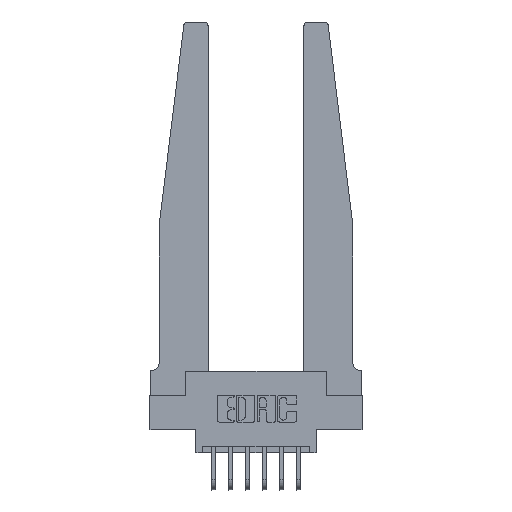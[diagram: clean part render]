
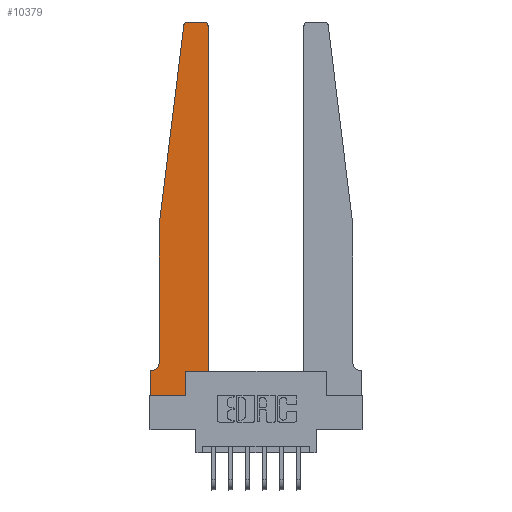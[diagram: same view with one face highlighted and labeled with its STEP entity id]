
A CAD part, top view. The second image highlights one B-rep face of the part: STEP entity #10379.
In plain terms, the highlighted planar face has unit normal (0, 0, 1).
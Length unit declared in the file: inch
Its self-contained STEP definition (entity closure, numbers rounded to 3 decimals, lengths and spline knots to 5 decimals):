
#15 = EDGE_CURVE ( 'NONE', #51, #5024, #1532, .T. ) ;
#51 = VERTEX_POINT ( 'NONE', #466 ) ;
#75 = DIRECTION ( 'NONE',  ( 0., 0., 1. ) ) ;
#79 = AXIS2_PLACEMENT_3D ( 'NONE', #8297, #8222, #9416 ) ;
#265 = DIRECTION ( 'NONE',  ( 0., -1., 0. ) ) ;
#386 = CARTESIAN_POINT ( 'NONE',  ( 0., 0.1875, 0.37 ) ) ;
#466 = CARTESIAN_POINT ( 'NONE',  ( 0.425, 0.18, 0.37 ) ) ;
#629 = LINE ( 'NONE', #7001, #10541 ) ;
#1075 = VECTOR ( 'NONE', #4248, 39.37008 ) ;
#1297 = AXIS2_PLACEMENT_3D ( 'NONE', #386, #4987, #5820 ) ;
#1425 = VERTEX_POINT ( 'NONE', #1536 ) ;
#1460 = EDGE_CURVE ( 'NONE', #2933, #8866, #4866, .T. ) ;
#1509 = VECTOR ( 'NONE', #9149, 39.37008 ) ;
#1532 = LINE ( 'NONE', #10071, #1509 ) ;
#1536 = CARTESIAN_POINT ( 'NONE',  ( 0.2605, 0., 0.37 ) ) ;
#1804 = CARTESIAN_POINT ( 'NONE',  ( 0.395, 2.75, 0.37 ) ) ;
#2175 = ORIENTED_EDGE ( 'NONE', *, *, #1460, .T. ) ;
#2325 = DIRECTION ( 'NONE',  ( 1., 0., 0. ) ) ;
#2933 = VERTEX_POINT ( 'NONE', #6547 ) ;
#3113 = DIRECTION ( 'NONE',  ( 1., 0., 0. ) ) ;
#3441 = EDGE_CURVE ( 'NONE', #8767, #4837, #9859, .T. ) ;
#3532 = VERTEX_POINT ( 'NONE', #3998 ) ;
#3546 = ORIENTED_EDGE ( 'NONE', *, *, #7056, .T. ) ;
#3662 = VECTOR ( 'NONE', #10256, 39.37008 ) ;
#3867 = DIRECTION ( 'NONE',  ( -1., 0., 0. ) ) ;
#3877 = VERTEX_POINT ( 'NONE', #13833 ) ;
#3893 = ORIENTED_EDGE ( 'NONE', *, *, #12143, .T. ) ;
#3950 = DIRECTION ( 'NONE',  ( 0., 1., 0. ) ) ;
#3998 = CARTESIAN_POINT ( 'NONE',  ( 0., 0., 0.37 ) ) ;
#4248 = DIRECTION ( 'NONE',  ( 0., -1., 0. ) ) ;
#4566 = EDGE_CURVE ( 'NONE', #3532, #1425, #10425, .T. ) ;
#4633 = EDGE_CURVE ( 'NONE', #8866, #3877, #13142, .T. ) ;
#4666 = CARTESIAN_POINT ( 'NONE',  ( 0.065, 1.25, 0.37 ) ) ;
#4837 = VERTEX_POINT ( 'NONE', #11630 ) ;
#4852 = ORIENTED_EDGE ( 'NONE', *, *, #5114, .T. ) ;
#4866 = CIRCLE ( 'NONE', #7585, 0.05 ) ;
#4867 = ORIENTED_EDGE ( 'NONE', *, *, #5274, .T. ) ;
#4987 = DIRECTION ( 'NONE',  ( 0., 0., 1. ) ) ;
#5024 = VERTEX_POINT ( 'NONE', #9045 ) ;
#5089 = CARTESIAN_POINT ( 'NONE',  ( 0., 0., 0.37 ) ) ;
#5114 = EDGE_CURVE ( 'NONE', #11187, #2933, #13076, .T. ) ;
#5141 = LINE ( 'NONE', #8386, #8218 ) ;
#5274 = EDGE_CURVE ( 'NONE', #13540, #51, #5141, .T. ) ;
#5371 = LINE ( 'NONE', #10481, #1075 ) ;
#5707 = CARTESIAN_POINT ( 'NONE',  ( 0.2605, 0.18, 0.37 ) ) ;
#5820 = DIRECTION ( 'NONE',  ( 1., 0., 0. ) ) ;
#5920 = VECTOR ( 'NONE', #9040, 39.37008 ) ;
#5953 = PLANE ( 'NONE',  #1297 ) ;
#6389 = CARTESIAN_POINT ( 'NONE',  ( 0.015, 0.1875, 0.37 ) ) ;
#6547 = CARTESIAN_POINT ( 'NONE',  ( 0.065, 0.2375, 0.37 ) ) ;
#6562 = EDGE_CURVE ( 'NONE', #4837, #10525, #10422, .T. ) ;
#6652 = CARTESIAN_POINT ( 'NONE',  ( 0.065, 0.1875, 0.37 ) ) ;
#6802 = ORIENTED_EDGE ( 'NONE', *, *, #4566, .T. ) ;
#6851 = EDGE_LOOP ( 'NONE', ( #7783, #9383, #3893, #4852, #2175, #8043, #7351, #6802, #11281, #4867, #12086, #3546 ) ) ;
#7001 = CARTESIAN_POINT ( 'NONE',  ( 0.2605, 0.18, 0.37 ) ) ;
#7056 = EDGE_CURVE ( 'NONE', #5024, #8767, #11143, .T. ) ;
#7351 = ORIENTED_EDGE ( 'NONE', *, *, #10135, .T. ) ;
#7499 = CARTESIAN_POINT ( 'NONE',  ( 0.395, 2.72, 0.37 ) ) ;
#7585 = AXIS2_PLACEMENT_3D ( 'NONE', #9085, #9155, #3867 ) ;
#7783 = ORIENTED_EDGE ( 'NONE', *, *, #3441, .T. ) ;
#7931 = DIRECTION ( 'NONE',  ( -0.122, -0.992, 0. ) ) ;
#8043 = ORIENTED_EDGE ( 'NONE', *, *, #4633, .T. ) ;
#8218 = VECTOR ( 'NONE', #12691, 39.37008 ) ;
#8222 = DIRECTION ( 'NONE',  ( 0., 0., 1. ) ) ;
#8297 = CARTESIAN_POINT ( 'NONE',  ( 0.27653, 2.72, 0.37 ) ) ;
#8386 = CARTESIAN_POINT ( 'NONE',  ( 0.425, 0.18, 0.37 ) ) ;
#8767 = VERTEX_POINT ( 'NONE', #1804 ) ;
#8866 = VERTEX_POINT ( 'NONE', #6389 ) ;
#8876 = VECTOR ( 'NONE', #265, 39.37008 ) ;
#8892 = CARTESIAN_POINT ( 'NONE',  ( 0.065, 1.25, 0.37 ) ) ;
#9040 = DIRECTION ( 'NONE',  ( -1., 0., 0. ) ) ;
#9045 = CARTESIAN_POINT ( 'NONE',  ( 0.425, 2.72, 0.37 ) ) ;
#9082 = VECTOR ( 'NONE', #3113, 39.37008 ) ;
#9085 = CARTESIAN_POINT ( 'NONE',  ( 0.015, 0.2375, 0.37 ) ) ;
#9149 = DIRECTION ( 'NONE',  ( 0., 1., 0. ) ) ;
#9155 = DIRECTION ( 'NONE',  ( 0., 0., -1. ) ) ;
#9383 = ORIENTED_EDGE ( 'NONE', *, *, #6562, .T. ) ;
#9416 = DIRECTION ( 'NONE',  ( 1., 0., 0. ) ) ;
#9447 = VECTOR ( 'NONE', #7931, 39.37008 ) ;
#9859 = LINE ( 'NONE', #13663, #3662 ) ;
#10071 = CARTESIAN_POINT ( 'NONE',  ( 0.425, 0.18, 0.37 ) ) ;
#10135 = EDGE_CURVE ( 'NONE', #3877, #3532, #5371, .T. ) ;
#10256 = DIRECTION ( 'NONE',  ( -1., 0., 0. ) ) ;
#10379 = ADVANCED_FACE ( 'NONE', ( #12256 ), #5953, .T. ) ;
#10422 = CIRCLE ( 'NONE', #79, 0.03 ) ;
#10425 = LINE ( 'NONE', #5089, #9082 ) ;
#10436 = AXIS2_PLACEMENT_3D ( 'NONE', #7499, #75, #2325 ) ;
#10468 = CARTESIAN_POINT ( 'NONE',  ( 0.24675, 2.72367, 0.37 ) ) ;
#10481 = CARTESIAN_POINT ( 'NONE',  ( 0., 0., 0.37 ) ) ;
#10525 = VERTEX_POINT ( 'NONE', #10468 ) ;
#10541 = VECTOR ( 'NONE', #3950, 39.37008 ) ;
#11143 = CIRCLE ( 'NONE', #10436, 0.03 ) ;
#11187 = VERTEX_POINT ( 'NONE', #11267 ) ;
#11267 = CARTESIAN_POINT ( 'NONE',  ( 0.065, 1.25, 0.37 ) ) ;
#11281 = ORIENTED_EDGE ( 'NONE', *, *, #13729, .T. ) ;
#11630 = CARTESIAN_POINT ( 'NONE',  ( 0.27653, 2.75, 0.37 ) ) ;
#12023 = LINE ( 'NONE', #4666, #9447 ) ;
#12086 = ORIENTED_EDGE ( 'NONE', *, *, #15, .T. ) ;
#12143 = EDGE_CURVE ( 'NONE', #10525, #11187, #12023, .T. ) ;
#12256 = FACE_OUTER_BOUND ( 'NONE', #6851, .T. ) ;
#12691 = DIRECTION ( 'NONE',  ( 1., 0., 0. ) ) ;
#13076 = LINE ( 'NONE', #8892, #8876 ) ;
#13142 = LINE ( 'NONE', #6652, #5920 ) ;
#13540 = VERTEX_POINT ( 'NONE', #5707 ) ;
#13663 = CARTESIAN_POINT ( 'NONE',  ( 0.25, 2.75, 0.37 ) ) ;
#13729 = EDGE_CURVE ( 'NONE', #1425, #13540, #629, .T. ) ;
#13833 = CARTESIAN_POINT ( 'NONE',  ( 0., 0.1875, 0.37 ) ) ;
